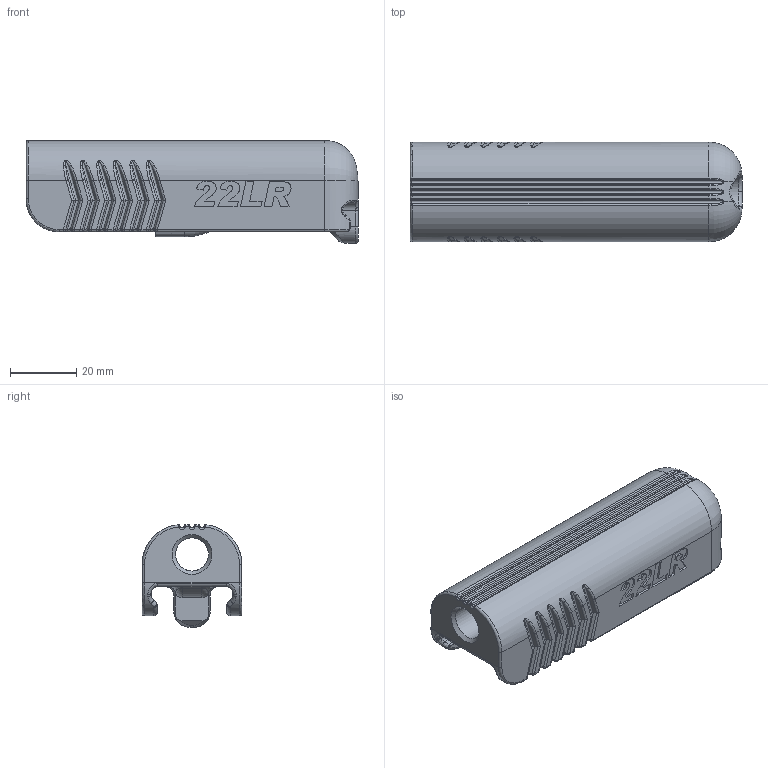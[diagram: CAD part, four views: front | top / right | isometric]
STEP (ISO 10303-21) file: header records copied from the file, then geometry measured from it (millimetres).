
FILE_DESCRIPTION(('FreeCAD Model'),'2;1');
FILE_NAME('Open CASCADE Shape Model','2022-12-07T11:22:42',('Author'),( ''),'Open CASCADE STEP processor 7.6','FreeCAD','Unknown');
FILE_SCHEMA(('AUTOMOTIVE_DESIGN { 1 0 10303 214 1 1 1 1 }'));
Length unit declared in the file: millimetre
Products named in the file (1): Slide
Bounding box: 100 x 30 x 31 mm (x, y, z)
Volume: 51316.5 mm3; surface area: 17543.7 mm2
Topology: 1 solids, 1 shells, 622 faces, 1556 edges, 944 vertices
Faces by surface type: bspline 187, cylinder 165, plane 155, extrusion 86, torus 25, cone 2, revolution 2
Full cylindrical faces by diameter (mm): 2 x1, 10 x1
Entity records: 79177 total; most frequent: CARTESIAN_POINT 52714, DIRECTION 3422, ORIENTED_EDGE 3112, PCURVE 3112, DEFINITIONAL_REPRESENTATION 3112, VECTOR 2331, LINE 2245, B_SPLINE_CURVE_WITH_KNOTS 1818
